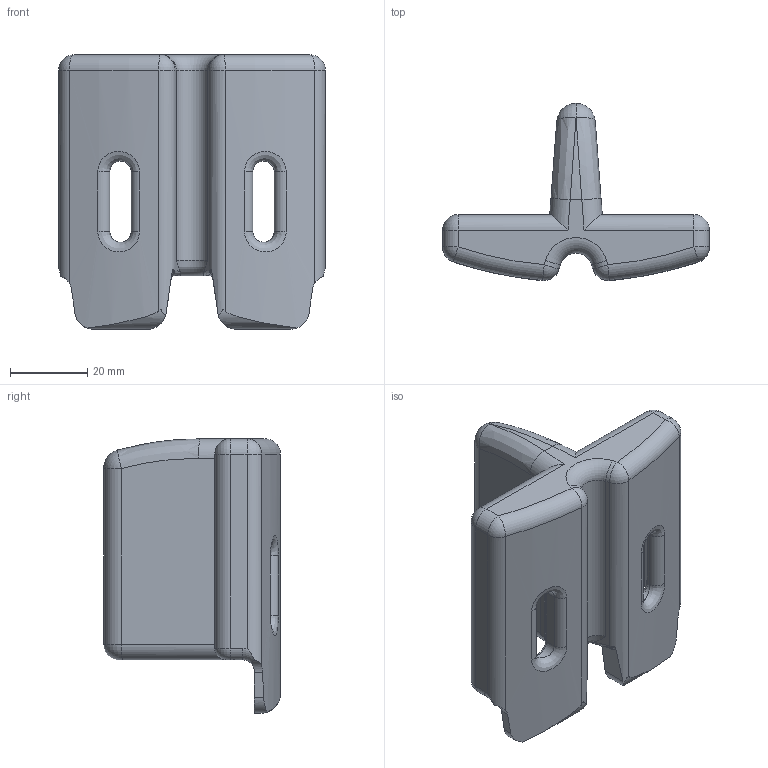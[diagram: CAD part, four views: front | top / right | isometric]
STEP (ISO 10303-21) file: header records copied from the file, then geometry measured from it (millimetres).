
FILE_DESCRIPTION (( 'STEP AP214' ), '1' );
FILE_NAME ('PmagM3Coupler3.STEP', '2020-02-26T02:10:19', ( '' ), ( '' ), 'SwSTEP 2.0', 'SolidWorks 2019', '' );
FILE_SCHEMA (( 'AUTOMOTIVE_DESIGN' ));
Length unit declared in the file: millimetre
Products named in the file (1): PmagM3Coupler3
Bounding box: 69 x 45.79 x 71 mm (x, y, z)
Volume: 48461.7 mm3; surface area: 18997.8 mm2
Topology: 1 solids, 1 shells, 183 faces, 466 edges, 281 vertices
Faces by surface type: plane 83, cylinder 63, torus 15, bspline 14, sphere 8
Entity records: 7663 total; most frequent: CARTESIAN_POINT 2515, ORIENTED_EDGE 924, DIRECTION 797, EDGE_CURVE 462, VERTEX_POINT 281, AXIS2_PLACEMENT_3D 272, LINE 253, VECTOR 253
